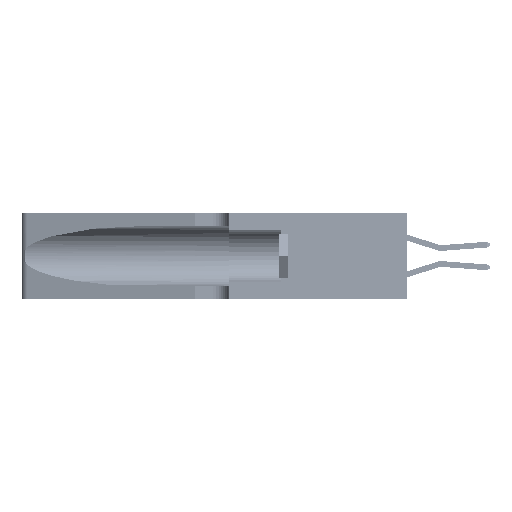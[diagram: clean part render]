
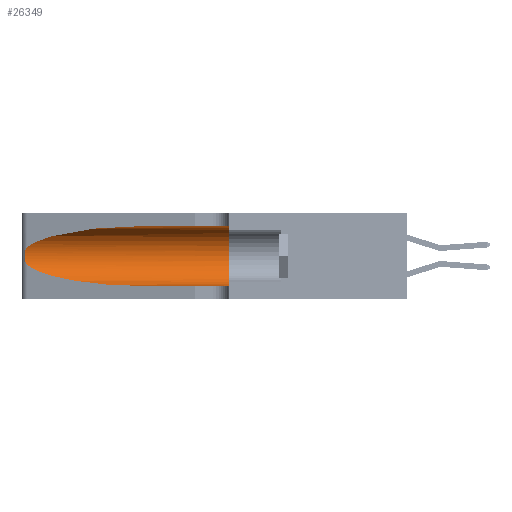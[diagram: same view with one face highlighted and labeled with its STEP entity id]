
A CAD part, left-side view. The second image highlights one B-rep face of the part: STEP entity #26349.
In plain terms, the highlighted cylindrical face has radius 3.308 mm (diameter 6.617 mm), a partial arc.
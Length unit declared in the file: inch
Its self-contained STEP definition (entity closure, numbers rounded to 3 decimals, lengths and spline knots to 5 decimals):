
#844 = DIRECTION ( 'NONE',  ( 0., 0., -1. ) ) ;
#1563 = ORIENTED_EDGE ( 'NONE', *, *, #25180, .T. ) ;
#1993 = DIRECTION ( 'NONE',  ( 0., -1., 0. ) ) ;
#3663 = CARTESIAN_POINT ( 'NONE',  ( 0.26018, 1.23835, 0.19895 ) ) ;
#4423 = CARTESIAN_POINT ( 'NONE',  ( 0.25487, 1.22718, 0.22369 ) ) ;
#6156 = AXIS2_PLACEMENT_3D ( 'NONE', #51634, #22284, #844 ) ;
#7212 = EDGE_CURVE ( 'NONE', #35965, #37743, #43506, .T. ) ;
#7996 = CARTESIAN_POINT ( 'NONE',  ( 0.26075, 1.23896, 0.178 ) ) ;
#9131 = ORIENTED_EDGE ( 'NONE', *, *, #46164, .T. ) ;
#10476 = CYLINDRICAL_SURFACE ( 'NONE', #6156, 0.13025 ) ;
#11683 = EDGE_CURVE ( 'NONE', #45493, #37743, #49491, .T. ) ;
#12304 = CARTESIAN_POINT ( 'NONE',  ( 0.25856, 1.23593, 0.16098 ) ) ;
#13010 = VERTEX_POINT ( 'NONE', #38392 ) ;
#14518 = CARTESIAN_POINT ( 'NONE',  ( 0.2373, 1.15595, 0.28018 ) ) ;
#16626 = CARTESIAN_POINT ( 'NONE',  ( 0.25487, 1.22718, 0.14631 ) ) ;
#16693 = CARTESIAN_POINT ( 'NONE',  ( 0.25639, 1.23186, 0.15144 ) ) ;
#20510 = AXIS2_PLACEMENT_3D ( 'NONE', #24369, #53715, #28634 ) ;
#20868 = VERTEX_POINT ( 'NONE', #4423 ) ;
#20911 = CARTESIAN_POINT ( 'NONE',  ( 0.2373, 1.15595, 0.08982 ) ) ;
#20974 = CARTESIAN_POINT ( 'NONE',  ( 0.25487, 1.22718, 0.14631 ) ) ;
#22284 = DIRECTION ( 'NONE',  ( 0., -1., 0. ) ) ;
#22897 =( BOUNDED_CURVE ( )  B_SPLINE_CURVE ( 3, ( #16626, #20911, #50281, #25150 ),
 .UNSPECIFIED., .F., .T. ) 
 B_SPLINE_CURVE_WITH_KNOTS ( ( 4, 4 ),
 ( 3.44316, 4.71239 ),
 .UNSPECIFIED. ) 
 CURVE ( )  GEOMETRIC_REPRESENTATION_ITEM ( )  RATIONAL_B_SPLINE_CURVE ( ( 1., 0.87, 0.87, 1. ) ) 
 REPRESENTATION_ITEM ( '' )  );
#23402 = CARTESIAN_POINT ( 'NONE',  ( 0.1305, 1.61858, 0.31525 ) ) ;
#23409 = CARTESIAN_POINT ( 'NONE',  ( 0.1305, 0.72297, 0.05475 ) ) ;
#24256 = ORIENTED_EDGE ( 'NONE', *, *, #34272, .T. ) ;
#24369 = CARTESIAN_POINT ( 'NONE',  ( 0.1305, 0.35, 0.185 ) ) ;
#25039 = CARTESIAN_POINT ( 'NONE',  ( 0.25639, 1.23184, 0.21858 ) ) ;
#25150 = CARTESIAN_POINT ( 'NONE',  ( 0.1305, 0.72297, 0.05475 ) ) ;
#25180 = EDGE_CURVE ( 'NONE', #27036, #20868, #26943, .T. ) ;
#26349 = ADVANCED_FACE ( 'NONE', ( #44273 ), #10476, .F. ) ;
#26943 =( BOUNDED_CURVE ( )  B_SPLINE_CURVE ( 3, ( #31439, #43899, #14518, #44072 ),
 .UNSPECIFIED., .F., .T. ) 
 B_SPLINE_CURVE_WITH_KNOTS ( ( 4, 4 ),
 ( 1.5708, 2.84003 ),
 .UNSPECIFIED. ) 
 CURVE ( )  GEOMETRIC_REPRESENTATION_ITEM ( )  RATIONAL_B_SPLINE_CURVE ( ( 1., 0.87, 0.87, 1. ) ) 
 REPRESENTATION_ITEM ( '' )  );
#27036 = VERTEX_POINT ( 'NONE', #35501 ) ;
#28634 = DIRECTION ( 'NONE',  ( 0., 0., 1. ) ) ;
#28828 = EDGE_CURVE ( 'NONE', #27036, #45493, #45377, .T. ) ;
#29294 = CARTESIAN_POINT ( 'NONE',  ( 0.25854, 1.2359, 0.20912 ) ) ;
#31439 = CARTESIAN_POINT ( 'NONE',  ( 0.1305, 0.72297, 0.31525 ) ) ;
#33546 = CARTESIAN_POINT ( 'NONE',  ( 0.26075, 1.23896, 0.19203 ) ) ;
#34068 = ORIENTED_EDGE ( 'NONE', *, *, #11683, .F. ) ;
#34245 = CARTESIAN_POINT ( 'NONE',  ( 0.1305, 1.61858, 0.05475 ) ) ;
#34272 = EDGE_CURVE ( 'NONE', #20868, #13010, #52146, .T. ) ;
#34289 = VECTOR ( 'NONE', #1993, 39.37008 ) ;
#35501 = CARTESIAN_POINT ( 'NONE',  ( 0.1305, 0.72297, 0.31525 ) ) ;
#35965 = VERTEX_POINT ( 'NONE', #23409 ) ;
#36130 = CARTESIAN_POINT ( 'NONE',  ( 0.1305, 0.35, 0.31525 ) ) ;
#37743 = VERTEX_POINT ( 'NONE', #45389 ) ;
#37758 = CARTESIAN_POINT ( 'NONE',  ( 0.26017, 1.23833, 0.17102 ) ) ;
#38392 = CARTESIAN_POINT ( 'NONE',  ( 0.25487, 1.22718, 0.14631 ) ) ;
#40603 = EDGE_LOOP ( 'NONE', ( #1563, #24256, #9131, #54472, #34068, #50349 ) ) ;
#41944 = CARTESIAN_POINT ( 'NONE',  ( 0.25789, 1.23486, 0.15765 ) ) ;
#42198 = VECTOR ( 'NONE', #46824, 39.37008 ) ;
#43506 = LINE ( 'NONE', #34245, #42198 ) ;
#43899 = CARTESIAN_POINT ( 'NONE',  ( 0.18966, 0.96281, 0.31525 ) ) ;
#44072 = CARTESIAN_POINT ( 'NONE',  ( 0.25487, 1.22718, 0.22369 ) ) ;
#44273 = FACE_OUTER_BOUND ( 'NONE', #40603, .T. ) ;
#45377 = LINE ( 'NONE', #23402, #34289 ) ;
#45389 = CARTESIAN_POINT ( 'NONE',  ( 0.1305, 0.35, 0.05475 ) ) ;
#45493 = VERTEX_POINT ( 'NONE', #36130 ) ;
#45972 = CARTESIAN_POINT ( 'NONE',  ( 0.25487, 1.22718, 0.22369 ) ) ;
#46147 = CARTESIAN_POINT ( 'NONE',  ( 0.25555, 1.22993, 0.14849 ) ) ;
#46164 = EDGE_CURVE ( 'NONE', #13010, #35965, #22897, .T. ) ;
#46824 = DIRECTION ( 'NONE',  ( 0., -1., 0. ) ) ;
#49491 = CIRCLE ( 'NONE', #20510, 0.13025 ) ;
#50161 = CARTESIAN_POINT ( 'NONE',  ( 0.25555, 1.22994, 0.2215 ) ) ;
#50281 = CARTESIAN_POINT ( 'NONE',  ( 0.18966, 0.96281, 0.05475 ) ) ;
#50349 = ORIENTED_EDGE ( 'NONE', *, *, #28828, .F. ) ;
#51634 = CARTESIAN_POINT ( 'NONE',  ( 0.1305, 1.61858, 0.185 ) ) ;
#52146 = B_SPLINE_CURVE_WITH_KNOTS ( 'NONE', 3,
 ( #45972, #50161, #25039, #54368, #29294, #3663, #33546, #7996, #37758, #12304, #41944, #16693, #46147, #20974 ),
 .UNSPECIFIED., .F., .F.,
 ( 4, 2, 2, 2, 2, 2, 4 ),
 ( 0., 0.00027, 0.00053, 0.00107, 0.0016, 0.00187, 0.00214 ),
 .UNSPECIFIED. ) ;
#53715 = DIRECTION ( 'NONE',  ( 0., 1., 0. ) ) ;
#54368 = CARTESIAN_POINT ( 'NONE',  ( 0.25787, 1.23484, 0.2124 ) ) ;
#54472 = ORIENTED_EDGE ( 'NONE', *, *, #7212, .T. ) ;
